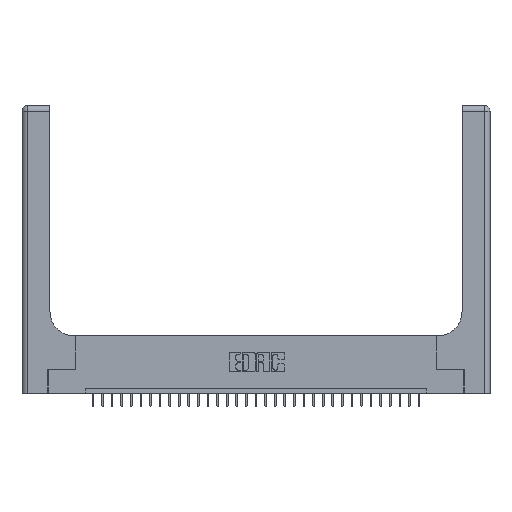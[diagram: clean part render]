
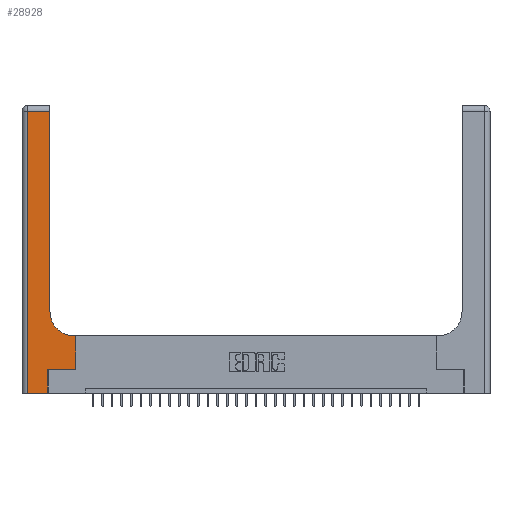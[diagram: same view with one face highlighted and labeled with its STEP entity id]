
A CAD part, top view. The second image highlights one B-rep face of the part: STEP entity #28928.
In plain terms, the highlighted planar face has unit normal (0, 0, 1).
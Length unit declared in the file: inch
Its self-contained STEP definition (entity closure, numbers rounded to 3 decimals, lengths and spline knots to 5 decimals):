
#662 = CARTESIAN_POINT ( 'NONE',  ( 0., 0., 0.37 ) ) ;
#1286 = VERTEX_POINT ( 'NONE', #4421 ) ;
#1596 = VECTOR ( 'NONE', #7139, 39.37008 ) ;
#1858 = ORIENTED_EDGE ( 'NONE', *, *, #32308, .T. ) ;
#2422 = CARTESIAN_POINT ( 'NONE',  ( 0.5585, 0.6, 0.37 ) ) ;
#2856 = CARTESIAN_POINT ( 'NONE',  ( 0.06, 0., 0.37 ) ) ;
#3340 = VECTOR ( 'NONE', #17342, 39.37008 ) ;
#3397 = CARTESIAN_POINT ( 'NONE',  ( 0.269, 0.25, 0.37 ) ) ;
#3890 = CARTESIAN_POINT ( 'NONE',  ( 0.269, 0., 0.37 ) ) ;
#3935 = CIRCLE ( 'NONE', #5023, 0.25 ) ;
#4421 = CARTESIAN_POINT ( 'NONE',  ( 0.269, 0., 0.37 ) ) ;
#5023 = AXIS2_PLACEMENT_3D ( 'NONE', #30231, #17859, #30391 ) ;
#5555 = EDGE_CURVE ( 'NONE', #31989, #13206, #22567, .T. ) ;
#6167 = VECTOR ( 'NONE', #18022, 39.37008 ) ;
#7139 = DIRECTION ( 'NONE',  ( 0., 1., 0. ) ) ;
#7155 = EDGE_CURVE ( 'NONE', #31982, #31290, #27808, .T. ) ;
#7581 = EDGE_CURVE ( 'NONE', #25477, #16861, #25114, .T. ) ;
#7938 = CARTESIAN_POINT ( 'NONE',  ( 0.269, 0.25, 0.37 ) ) ;
#8080 = CARTESIAN_POINT ( 'NONE',  ( 0.06, 3., 0.37 ) ) ;
#9187 = PLANE ( 'NONE',  #11261 ) ;
#9334 = DIRECTION ( 'NONE',  ( -1., 0., 0. ) ) ;
#9829 = FACE_OUTER_BOUND ( 'NONE', #30700, .T. ) ;
#9968 = ORIENTED_EDGE ( 'NONE', *, *, #28233, .T. ) ;
#10535 = CARTESIAN_POINT ( 'NONE',  ( 0.5415, 0.6, 0.37 ) ) ;
#10630 = EDGE_CURVE ( 'NONE', #13206, #25477, #12389, .T. ) ;
#11261 = AXIS2_PLACEMENT_3D ( 'NONE', #24797, #32233, #9334 ) ;
#12056 = CARTESIAN_POINT ( 'NONE',  ( 0.5585, 0.25, 0.37 ) ) ;
#12281 = DIRECTION ( 'NONE',  ( 0., 1., 0. ) ) ;
#12389 = LINE ( 'NONE', #12056, #1596 ) ;
#12705 = DIRECTION ( 'NONE',  ( 1., 0., 0. ) ) ;
#13206 = VERTEX_POINT ( 'NONE', #28013 ) ;
#13945 = DIRECTION ( 'NONE',  ( 0., 1., 0. ) ) ;
#14152 = ORIENTED_EDGE ( 'NONE', *, *, #7581, .T. ) ;
#14219 = ORIENTED_EDGE ( 'NONE', *, *, #5555, .T. ) ;
#14318 = ORIENTED_EDGE ( 'NONE', *, *, #25850, .T. ) ;
#15065 = VECTOR ( 'NONE', #30761, 39.37008 ) ;
#15586 = CARTESIAN_POINT ( 'NONE',  ( 0.2915, 2.94, 0.37 ) ) ;
#16514 = ORIENTED_EDGE ( 'NONE', *, *, #24071, .T. ) ;
#16861 = VERTEX_POINT ( 'NONE', #10535 ) ;
#17342 = DIRECTION ( 'NONE',  ( 1., 0., 0. ) ) ;
#17741 = CARTESIAN_POINT ( 'NONE',  ( 0., 2.94, 0.37 ) ) ;
#17859 = DIRECTION ( 'NONE',  ( 0., 0., -1. ) ) ;
#18022 = DIRECTION ( 'NONE',  ( -1., 0., 0. ) ) ;
#19440 = ORIENTED_EDGE ( 'NONE', *, *, #7155, .T. ) ;
#20353 = CARTESIAN_POINT ( 'NONE',  ( 0.2915, 0.85, 0.37 ) ) ;
#21345 = LINE ( 'NONE', #3890, #28486 ) ;
#21729 = VERTEX_POINT ( 'NONE', #20353 ) ;
#22428 = CARTESIAN_POINT ( 'NONE',  ( 0.06, 2.94, 0.37 ) ) ;
#22567 = LINE ( 'NONE', #7938, #29302 ) ;
#24071 = EDGE_CURVE ( 'NONE', #31290, #24279, #30945, .T. ) ;
#24279 = VERTEX_POINT ( 'NONE', #2856 ) ;
#24797 = CARTESIAN_POINT ( 'NONE',  ( 0., 3., 0.37 ) ) ;
#25114 = LINE ( 'NONE', #30721, #6167 ) ;
#25477 = VERTEX_POINT ( 'NONE', #2422 ) ;
#25850 = EDGE_CURVE ( 'NONE', #1286, #31989, #21345, .T. ) ;
#26952 = LINE ( 'NONE', #27106, #28348 ) ;
#27106 = CARTESIAN_POINT ( 'NONE',  ( 0.2915, 3., 0.37 ) ) ;
#27340 = ORIENTED_EDGE ( 'NONE', *, *, #30256, .T. ) ;
#27405 = LINE ( 'NONE', #662, #3340 ) ;
#27808 = LINE ( 'NONE', #17741, #15065 ) ;
#28013 = CARTESIAN_POINT ( 'NONE',  ( 0.5585, 0.25, 0.37 ) ) ;
#28159 = DIRECTION ( 'NONE',  ( 0., -1., 0. ) ) ;
#28233 = EDGE_CURVE ( 'NONE', #24279, #1286, #27405, .T. ) ;
#28348 = VECTOR ( 'NONE', #12281, 39.37008 ) ;
#28486 = VECTOR ( 'NONE', #13945, 39.37008 ) ;
#28928 = ADVANCED_FACE ( 'NONE', ( #9829 ), #9187, .F. ) ;
#29302 = VECTOR ( 'NONE', #12705, 39.37008 ) ;
#30231 = CARTESIAN_POINT ( 'NONE',  ( 0.5415, 0.85, 0.37 ) ) ;
#30256 = EDGE_CURVE ( 'NONE', #16861, #21729, #3935, .T. ) ;
#30287 = ORIENTED_EDGE ( 'NONE', *, *, #10630, .T. ) ;
#30391 = DIRECTION ( 'NONE',  ( 1., 0., 0. ) ) ;
#30700 = EDGE_LOOP ( 'NONE', ( #1858, #19440, #16514, #9968, #14318, #14219, #30287, #14152, #27340 ) ) ;
#30721 = CARTESIAN_POINT ( 'NONE',  ( 0.2915, 0.6, 0.37 ) ) ;
#30761 = DIRECTION ( 'NONE',  ( -1., 0., 0. ) ) ;
#30945 = LINE ( 'NONE', #8080, #31108 ) ;
#31108 = VECTOR ( 'NONE', #28159, 39.37008 ) ;
#31290 = VERTEX_POINT ( 'NONE', #22428 ) ;
#31982 = VERTEX_POINT ( 'NONE', #15586 ) ;
#31989 = VERTEX_POINT ( 'NONE', #3397 ) ;
#32233 = DIRECTION ( 'NONE',  ( 0., 0., -1. ) ) ;
#32308 = EDGE_CURVE ( 'NONE', #21729, #31982, #26952, .T. ) ;
